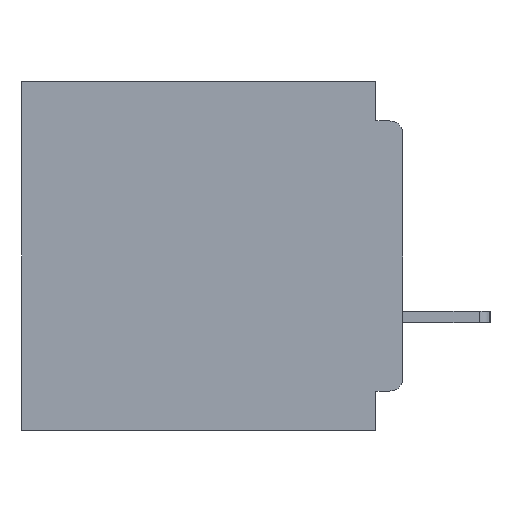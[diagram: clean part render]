
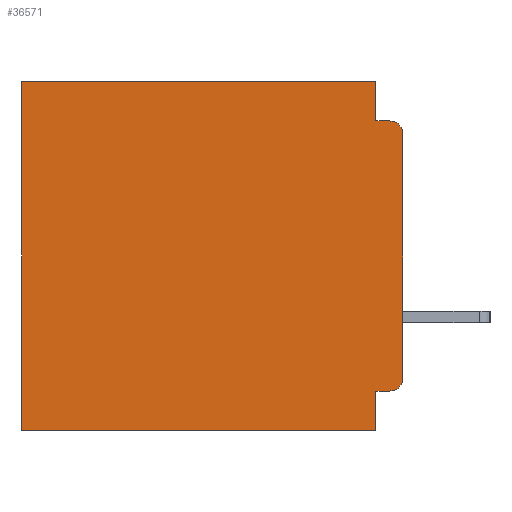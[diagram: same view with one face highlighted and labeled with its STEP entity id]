
A CAD part, left-side view. The second image highlights one B-rep face of the part: STEP entity #36571.
In plain terms, the highlighted planar face has unit normal (-1, 0, 0).
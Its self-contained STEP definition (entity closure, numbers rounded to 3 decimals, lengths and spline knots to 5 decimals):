
#603 = ORIENTED_EDGE ( 'NONE', *, *, #40675, .F. ) ;
#1579 = VERTEX_POINT ( 'NONE', #50292 ) ;
#1629 = VERTEX_POINT ( 'NONE', #30327 ) ;
#3382 = EDGE_CURVE ( 'NONE', #7975, #1579, #31311, .T. ) ;
#3564 = CARTESIAN_POINT ( 'NONE',  ( 0.3, 0., -0.4 ) ) ;
#4959 = VECTOR ( 'NONE', #54660, 39.37008 ) ;
#6653 = DIRECTION ( 'NONE',  ( 0., 0., -1. ) ) ;
#7975 = VERTEX_POINT ( 'NONE', #37110 ) ;
#8377 = CARTESIAN_POINT ( 'NONE',  ( 0.3, 0.031, -0.4 ) ) ;
#8827 = VECTOR ( 'NONE', #17730, 39.37008 ) ;
#8894 = CARTESIAN_POINT ( 'NONE',  ( 0.3, 0.015, -0.045 ) ) ;
#9289 = EDGE_CURVE ( 'NONE', #50328, #48462, #26496, .T. ) ;
#10139 = VECTOR ( 'NONE', #6653, 39.37008 ) ;
#13644 = AXIS2_PLACEMENT_3D ( 'NONE', #53871, #58370, #31181 ) ;
#14159 = VECTOR ( 'NONE', #36392, 39.37008 ) ;
#14562 = LINE ( 'NONE', #20568, #10139 ) ;
#15032 = CARTESIAN_POINT ( 'NONE',  ( 0.3, 0.015, -0.06 ) ) ;
#15191 = ORIENTED_EDGE ( 'NONE', *, *, #52383, .T. ) ;
#15972 = LINE ( 'NONE', #18316, #4959 ) ;
#16407 = DIRECTION ( 'NONE',  ( 0., 0., -1. ) ) ;
#17069 = CARTESIAN_POINT ( 'NONE',  ( 0.3, 0.437, -0.4 ) ) ;
#17177 = CARTESIAN_POINT ( 'NONE',  ( 0.3, 0.031, -0.355 ) ) ;
#17730 = DIRECTION ( 'NONE',  ( 0., 1., 0. ) ) ;
#17843 = CARTESIAN_POINT ( 'NONE',  ( 0.3, 0.031, -0.4 ) ) ;
#18223 = CARTESIAN_POINT ( 'NONE',  ( 0.3, 0.031, 0. ) ) ;
#18316 = CARTESIAN_POINT ( 'NONE',  ( 0.3, 0., -0.355 ) ) ;
#19713 = DIRECTION ( 'NONE',  ( 0., 0., -1. ) ) ;
#20568 = CARTESIAN_POINT ( 'NONE',  ( 0.3, 0., -0.4 ) ) ;
#20607 = VECTOR ( 'NONE', #49124, 39.37008 ) ;
#20896 = ORIENTED_EDGE ( 'NONE', *, *, #3382, .T. ) ;
#22173 = DIRECTION ( 'NONE',  ( 0., 1., 0. ) ) ;
#22833 = ORIENTED_EDGE ( 'NONE', *, *, #38364, .T. ) ;
#23328 = AXIS2_PLACEMENT_3D ( 'NONE', #52971, #53801, #58955 ) ;
#25540 = CARTESIAN_POINT ( 'NONE',  ( 0.3, 0.031, 0. ) ) ;
#26487 = LINE ( 'NONE', #17843, #14159 ) ;
#26496 = LINE ( 'NONE', #47360, #52162 ) ;
#26759 = ORIENTED_EDGE ( 'NONE', *, *, #47220, .F. ) ;
#30024 = ORIENTED_EDGE ( 'NONE', *, *, #9289, .F. ) ;
#30327 = CARTESIAN_POINT ( 'NONE',  ( 0.3, 0.437, 0. ) ) ;
#31181 = DIRECTION ( 'NONE',  ( 0., 0., -1. ) ) ;
#31311 = CIRCLE ( 'NONE', #23328, 0.015 ) ;
#31652 = EDGE_LOOP ( 'NONE', ( #33557, #53721, #30024, #603, #15191, #22833, #52498, #26759, #54606, #20896 ) ) ;
#31943 = CARTESIAN_POINT ( 'NONE',  ( 0.3, 0., -0.06 ) ) ;
#32050 = VERTEX_POINT ( 'NONE', #31943 ) ;
#33499 = AXIS2_PLACEMENT_3D ( 'NONE', #15032, #47120, #19713 ) ;
#33557 = ORIENTED_EDGE ( 'NONE', *, *, #52166, .F. ) ;
#33980 = VERTEX_POINT ( 'NONE', #18223 ) ;
#34983 = LINE ( 'NONE', #3564, #8827 ) ;
#35454 = VECTOR ( 'NONE', #16407, 39.37008 ) ;
#36392 = DIRECTION ( 'NONE',  ( 0., 0., -1. ) ) ;
#36571 = ADVANCED_FACE ( 'NONE', ( #50858 ), #49320, .F. ) ;
#37110 = CARTESIAN_POINT ( 'NONE',  ( 0.3, 0.015, -0.355 ) ) ;
#37800 = CARTESIAN_POINT ( 'NONE',  ( 0.3, 0.031, -0.045 ) ) ;
#38364 = EDGE_CURVE ( 'NONE', #1629, #52309, #56971, .T. ) ;
#40675 = EDGE_CURVE ( 'NONE', #33980, #50328, #48942, .T. ) ;
#45787 = VERTEX_POINT ( 'NONE', #17177 ) ;
#46131 = VECTOR ( 'NONE', #22173, 39.37008 ) ;
#46969 = DIRECTION ( 'NONE',  ( 0., -1., 0. ) ) ;
#47120 = DIRECTION ( 'NONE',  ( -1., 0., 0. ) ) ;
#47220 = EDGE_CURVE ( 'NONE', #45787, #57566, #26487, .T. ) ;
#47267 = CIRCLE ( 'NONE', #33499, 0.015 ) ;
#47360 = CARTESIAN_POINT ( 'NONE',  ( 0.3, 0., -0.045 ) ) ;
#47543 = LINE ( 'NONE', #58385, #46131 ) ;
#48381 = EDGE_CURVE ( 'NONE', #57566, #52309, #34983, .T. ) ;
#48462 = VERTEX_POINT ( 'NONE', #8894 ) ;
#48942 = LINE ( 'NONE', #25540, #35454 ) ;
#49124 = DIRECTION ( 'NONE',  ( 0., 0., -1. ) ) ;
#49142 = CARTESIAN_POINT ( 'NONE',  ( 0.3, 0.437, -0.4 ) ) ;
#49320 = PLANE ( 'NONE',  #13644 ) ;
#50292 = CARTESIAN_POINT ( 'NONE',  ( 0.3, 0., -0.34 ) ) ;
#50328 = VERTEX_POINT ( 'NONE', #37800 ) ;
#50858 = FACE_OUTER_BOUND ( 'NONE', #31652, .T. ) ;
#52162 = VECTOR ( 'NONE', #46969, 39.37008 ) ;
#52166 = EDGE_CURVE ( 'NONE', #32050, #1579, #14562, .T. ) ;
#52309 = VERTEX_POINT ( 'NONE', #49142 ) ;
#52383 = EDGE_CURVE ( 'NONE', #33980, #1629, #47543, .T. ) ;
#52478 = EDGE_CURVE ( 'NONE', #7975, #45787, #15972, .T. ) ;
#52498 = ORIENTED_EDGE ( 'NONE', *, *, #48381, .F. ) ;
#52971 = CARTESIAN_POINT ( 'NONE',  ( 0.3, 0.015, -0.34 ) ) ;
#53721 = ORIENTED_EDGE ( 'NONE', *, *, #55134, .T. ) ;
#53801 = DIRECTION ( 'NONE',  ( -1., 0., 0. ) ) ;
#53871 = CARTESIAN_POINT ( 'NONE',  ( 0.3, 0., -0.4 ) ) ;
#54606 = ORIENTED_EDGE ( 'NONE', *, *, #52478, .F. ) ;
#54660 = DIRECTION ( 'NONE',  ( 0., 1., 0. ) ) ;
#55134 = EDGE_CURVE ( 'NONE', #32050, #48462, #47267, .T. ) ;
#56971 = LINE ( 'NONE', #17069, #20607 ) ;
#57566 = VERTEX_POINT ( 'NONE', #8377 ) ;
#58370 = DIRECTION ( 'NONE',  ( 1., 0., 0. ) ) ;
#58385 = CARTESIAN_POINT ( 'NONE',  ( 0.3, 0., 0. ) ) ;
#58955 = DIRECTION ( 'NONE',  ( 0., 0., -1. ) ) ;
